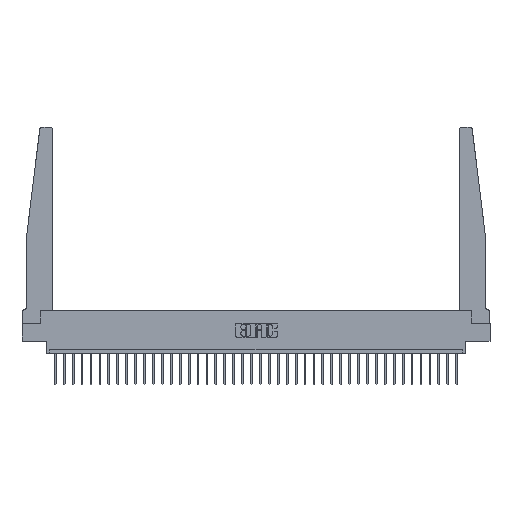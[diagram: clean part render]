
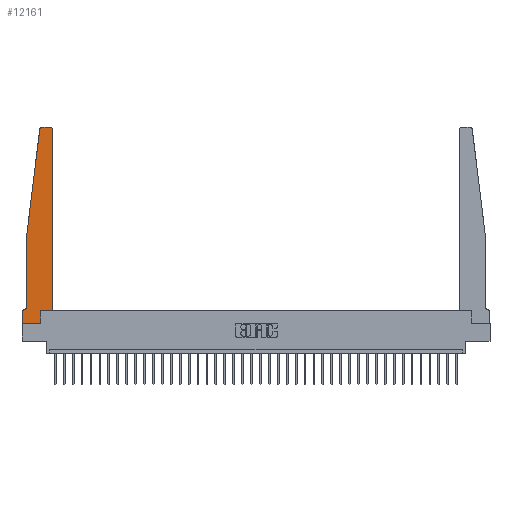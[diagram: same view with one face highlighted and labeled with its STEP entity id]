
A CAD part, top view. The second image highlights one B-rep face of the part: STEP entity #12161.
In plain terms, the highlighted planar face has unit normal (0, 0, 1).
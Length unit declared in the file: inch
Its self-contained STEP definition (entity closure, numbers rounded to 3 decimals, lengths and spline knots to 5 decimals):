
#158 = CIRCLE ( 'NONE', #28693, 0.05 ) ;
#480 = DIRECTION ( 'NONE',  ( 0., 0., 1. ) ) ;
#511 = EDGE_CURVE ( 'NONE', #23755, #27601, #5039, .T. ) ;
#668 = ORIENTED_EDGE ( 'NONE', *, *, #11469, .T. ) ;
#1638 = DIRECTION ( 'NONE',  ( 0., 0., -1. ) ) ;
#1747 = DIRECTION ( 'NONE',  ( -1., 0., 0. ) ) ;
#2237 = VECTOR ( 'NONE', #3410, 39.37008 ) ;
#2367 = LINE ( 'NONE', #16460, #16708 ) ;
#2484 = LINE ( 'NONE', #5769, #12053 ) ;
#3206 = FACE_OUTER_BOUND ( 'NONE', #15149, .T. ) ;
#3273 = LINE ( 'NONE', #16872, #17983 ) ;
#3312 = ORIENTED_EDGE ( 'NONE', *, *, #23244, .T. ) ;
#3410 = DIRECTION ( 'NONE',  ( 1., 0., 0. ) ) ;
#3922 = CARTESIAN_POINT ( 'NONE',  ( 0.065, 1.25, 0.37 ) ) ;
#4161 = DIRECTION ( 'NONE',  ( 0., -1., 0. ) ) ;
#4230 = EDGE_CURVE ( 'NONE', #25239, #8444, #21685, .T. ) ;
#4255 = VECTOR ( 'NONE', #9777, 39.37008 ) ;
#4369 = CARTESIAN_POINT ( 'NONE',  ( 0., 0., 0.37 ) ) ;
#4523 = CARTESIAN_POINT ( 'NONE',  ( 0.015, 0.2375, 0.37 ) ) ;
#4909 = DIRECTION ( 'NONE',  ( 0., 0., 1. ) ) ;
#5039 = CIRCLE ( 'NONE', #11901, 0.03 ) ;
#5375 = CARTESIAN_POINT ( 'NONE',  ( 0.395, 2.72, 0.37 ) ) ;
#5700 = VECTOR ( 'NONE', #14835, 39.37008 ) ;
#5769 = CARTESIAN_POINT ( 'NONE',  ( 0.065, 1.25, 0.37 ) ) ;
#6404 = EDGE_CURVE ( 'NONE', #16055, #25361, #23499, .T. ) ;
#6687 = CARTESIAN_POINT ( 'NONE',  ( 0.425, 0.18, 0.37 ) ) ;
#6786 = ORIENTED_EDGE ( 'NONE', *, *, #16164, .T. ) ;
#7360 = ORIENTED_EDGE ( 'NONE', *, *, #23813, .T. ) ;
#7768 = VECTOR ( 'NONE', #32328, 39.37008 ) ;
#7924 = ORIENTED_EDGE ( 'NONE', *, *, #14806, .T. ) ;
#8444 = VERTEX_POINT ( 'NONE', #9858 ) ;
#8481 = CARTESIAN_POINT ( 'NONE',  ( 0.395, 2.75, 0.37 ) ) ;
#9428 = CARTESIAN_POINT ( 'NONE',  ( 0.27653, 2.72, 0.37 ) ) ;
#9777 = DIRECTION ( 'NONE',  ( 1., 0., 0. ) ) ;
#9858 = CARTESIAN_POINT ( 'NONE',  ( 0.425, 2.72, 0.37 ) ) ;
#9918 = CARTESIAN_POINT ( 'NONE',  ( 0., 0.1875, 0.37 ) ) ;
#10038 = DIRECTION ( 'NONE',  ( 1., 0., 0. ) ) ;
#10805 = EDGE_CURVE ( 'NONE', #10965, #16055, #12505, .T. ) ;
#10965 = VERTEX_POINT ( 'NONE', #14414 ) ;
#11032 = VERTEX_POINT ( 'NONE', #3922 ) ;
#11469 = EDGE_CURVE ( 'NONE', #11032, #29698, #2484, .T. ) ;
#11901 = AXIS2_PLACEMENT_3D ( 'NONE', #9428, #24517, #29646 ) ;
#12053 = VECTOR ( 'NONE', #28404, 39.37008 ) ;
#12105 = VERTEX_POINT ( 'NONE', #8481 ) ;
#12161 = ADVANCED_FACE ( 'NONE', ( #3206 ), #19689, .T. ) ;
#12427 = VECTOR ( 'NONE', #4161, 39.37008 ) ;
#12505 = LINE ( 'NONE', #24894, #5700 ) ;
#12602 = CARTESIAN_POINT ( 'NONE',  ( 0., 0., 0.37 ) ) ;
#13867 = CIRCLE ( 'NONE', #17762, 0.03 ) ;
#14414 = CARTESIAN_POINT ( 'NONE',  ( 0.015, 0.1875, 0.37 ) ) ;
#14562 = EDGE_CURVE ( 'NONE', #25361, #21214, #31267, .T. ) ;
#14806 = EDGE_CURVE ( 'NONE', #15894, #25239, #19734, .T. ) ;
#14835 = DIRECTION ( 'NONE',  ( -1., 0., 0. ) ) ;
#15149 = EDGE_LOOP ( 'NONE', ( #3312, #17934, #7360, #668, #6786, #21207, #18702, #15343, #28556, #7924, #30602, #23731 ) ) ;
#15343 = ORIENTED_EDGE ( 'NONE', *, *, #14562, .T. ) ;
#15894 = VERTEX_POINT ( 'NONE', #31078 ) ;
#16055 = VERTEX_POINT ( 'NONE', #29067 ) ;
#16164 = EDGE_CURVE ( 'NONE', #29698, #10965, #158, .T. ) ;
#16460 = CARTESIAN_POINT ( 'NONE',  ( 0.2605, 0.18, 0.37 ) ) ;
#16546 = DIRECTION ( 'NONE',  ( -1., 0., 0. ) ) ;
#16610 = CARTESIAN_POINT ( 'NONE',  ( 0.065, 1.25, 0.37 ) ) ;
#16700 = CARTESIAN_POINT ( 'NONE',  ( 0.425, 0.18, 0.37 ) ) ;
#16708 = VECTOR ( 'NONE', #27394, 39.37008 ) ;
#16872 = CARTESIAN_POINT ( 'NONE',  ( 0.25, 2.75, 0.37 ) ) ;
#17762 = AXIS2_PLACEMENT_3D ( 'NONE', #5375, #480, #23358 ) ;
#17934 = ORIENTED_EDGE ( 'NONE', *, *, #511, .T. ) ;
#17983 = VECTOR ( 'NONE', #16546, 39.37008 ) ;
#18702 = ORIENTED_EDGE ( 'NONE', *, *, #6404, .T. ) ;
#19689 = PLANE ( 'NONE',  #22660 ) ;
#19734 = LINE ( 'NONE', #23736, #2237 ) ;
#19761 = CARTESIAN_POINT ( 'NONE',  ( 0., 0., 0.37 ) ) ;
#20609 = EDGE_CURVE ( 'NONE', #8444, #12105, #13867, .T. ) ;
#21207 = ORIENTED_EDGE ( 'NONE', *, *, #10805, .T. ) ;
#21214 = VERTEX_POINT ( 'NONE', #26028 ) ;
#21685 = LINE ( 'NONE', #16700, #7768 ) ;
#22660 = AXIS2_PLACEMENT_3D ( 'NONE', #9918, #4909, #10038 ) ;
#23244 = EDGE_CURVE ( 'NONE', #12105, #23755, #3273, .T. ) ;
#23358 = DIRECTION ( 'NONE',  ( 1., 0., 0. ) ) ;
#23499 = LINE ( 'NONE', #4369, #12427 ) ;
#23731 = ORIENTED_EDGE ( 'NONE', *, *, #20609, .T. ) ;
#23736 = CARTESIAN_POINT ( 'NONE',  ( 0.425, 0.18, 0.37 ) ) ;
#23755 = VERTEX_POINT ( 'NONE', #29013 ) ;
#23813 = EDGE_CURVE ( 'NONE', #27601, #11032, #31875, .T. ) ;
#24517 = DIRECTION ( 'NONE',  ( 0., 0., 1. ) ) ;
#24894 = CARTESIAN_POINT ( 'NONE',  ( 0.065, 0.1875, 0.37 ) ) ;
#25239 = VERTEX_POINT ( 'NONE', #6687 ) ;
#25361 = VERTEX_POINT ( 'NONE', #12602 ) ;
#25658 = EDGE_CURVE ( 'NONE', #21214, #15894, #2367, .T. ) ;
#26028 = CARTESIAN_POINT ( 'NONE',  ( 0.2605, 0., 0.37 ) ) ;
#26694 = VECTOR ( 'NONE', #27107, 39.37008 ) ;
#27107 = DIRECTION ( 'NONE',  ( -0.122, -0.992, 0. ) ) ;
#27394 = DIRECTION ( 'NONE',  ( 0., 1., 0. ) ) ;
#27601 = VERTEX_POINT ( 'NONE', #28187 ) ;
#28187 = CARTESIAN_POINT ( 'NONE',  ( 0.24675, 2.72367, 0.37 ) ) ;
#28404 = DIRECTION ( 'NONE',  ( 0., -1., 0. ) ) ;
#28556 = ORIENTED_EDGE ( 'NONE', *, *, #25658, .T. ) ;
#28693 = AXIS2_PLACEMENT_3D ( 'NONE', #4523, #1638, #1747 ) ;
#29013 = CARTESIAN_POINT ( 'NONE',  ( 0.27653, 2.75, 0.37 ) ) ;
#29067 = CARTESIAN_POINT ( 'NONE',  ( 0., 0.1875, 0.37 ) ) ;
#29646 = DIRECTION ( 'NONE',  ( 1., 0., 0. ) ) ;
#29698 = VERTEX_POINT ( 'NONE', #31757 ) ;
#30602 = ORIENTED_EDGE ( 'NONE', *, *, #4230, .T. ) ;
#31078 = CARTESIAN_POINT ( 'NONE',  ( 0.2605, 0.18, 0.37 ) ) ;
#31267 = LINE ( 'NONE', #19761, #4255 ) ;
#31757 = CARTESIAN_POINT ( 'NONE',  ( 0.065, 0.2375, 0.37 ) ) ;
#31875 = LINE ( 'NONE', #16610, #26694 ) ;
#32328 = DIRECTION ( 'NONE',  ( 0., 1., 0. ) ) ;
